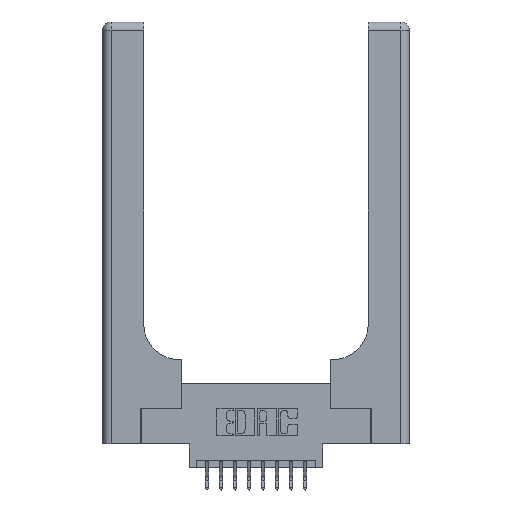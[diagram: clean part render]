
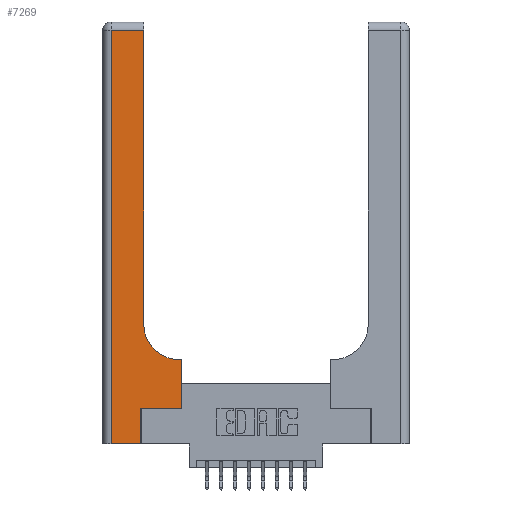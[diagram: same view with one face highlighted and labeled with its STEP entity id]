
A CAD part, top view. The second image highlights one B-rep face of the part: STEP entity #7269.
In plain terms, the highlighted planar face has unit normal (0, 0, 1).
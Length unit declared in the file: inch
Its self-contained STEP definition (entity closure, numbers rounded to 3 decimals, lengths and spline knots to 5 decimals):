
#210 = ORIENTED_EDGE ( 'NONE', *, *, #8994, .T. ) ;
#635 = CARTESIAN_POINT ( 'NONE',  ( 0.06, 0., 0.37 ) ) ;
#805 = EDGE_LOOP ( 'NONE', ( #210, #2820, #14824, #8057, #10947, #8593, #8192, #9050, #6819 ) ) ;
#823 = VERTEX_POINT ( 'NONE', #1749 ) ;
#869 = VERTEX_POINT ( 'NONE', #13013 ) ;
#1157 = CARTESIAN_POINT ( 'NONE',  ( 0.06, 3., 0.37 ) ) ;
#1540 = CARTESIAN_POINT ( 'NONE',  ( 0.269, 0.25, 0.37 ) ) ;
#1749 = CARTESIAN_POINT ( 'NONE',  ( 0.06, 2.94, 0.37 ) ) ;
#1825 = CARTESIAN_POINT ( 'NONE',  ( 0.269, 0.25, 0.37 ) ) ;
#2084 = CARTESIAN_POINT ( 'NONE',  ( 0.2915, 3., 0.37 ) ) ;
#2417 = DIRECTION ( 'NONE',  ( 1., 0., 0. ) ) ;
#2820 = ORIENTED_EDGE ( 'NONE', *, *, #3754, .T. ) ;
#2940 = VECTOR ( 'NONE', #7487, 39.37008 ) ;
#3478 = EDGE_CURVE ( 'NONE', #10670, #12525, #8065, .T. ) ;
#3628 = DIRECTION ( 'NONE',  ( -1., 0., 0. ) ) ;
#3647 = FACE_OUTER_BOUND ( 'NONE', #805, .T. ) ;
#3754 = EDGE_CURVE ( 'NONE', #12911, #823, #10224, .T. ) ;
#4066 = DIRECTION ( 'NONE',  ( -1., 0., 0. ) ) ;
#4224 = CARTESIAN_POINT ( 'NONE',  ( 0.269, 0., 0.37 ) ) ;
#4367 = VECTOR ( 'NONE', #3628, 39.37008 ) ;
#4794 = CARTESIAN_POINT ( 'NONE',  ( 0.2915, 0.6, 0.37 ) ) ;
#4896 = LINE ( 'NONE', #1157, #8446 ) ;
#5685 = VERTEX_POINT ( 'NONE', #9725 ) ;
#6125 = VECTOR ( 'NONE', #9954, 39.37008 ) ;
#6624 = DIRECTION ( 'NONE',  ( 0., 1., 0. ) ) ;
#6746 = CARTESIAN_POINT ( 'NONE',  ( 0., 2.94, 0.37 ) ) ;
#6755 = VECTOR ( 'NONE', #6624, 39.37008 ) ;
#6819 = ORIENTED_EDGE ( 'NONE', *, *, #9797, .T. ) ;
#7011 = DIRECTION ( 'NONE',  ( 0., 0., -1. ) ) ;
#7060 = CARTESIAN_POINT ( 'NONE',  ( 0.5585, 0.25, 0.37 ) ) ;
#7222 = DIRECTION ( 'NONE',  ( 0., 1., 0. ) ) ;
#7269 = ADVANCED_FACE ( 'NONE', ( #3647 ), #11799, .F. ) ;
#7487 = DIRECTION ( 'NONE',  ( 1., 0., 0. ) ) ;
#7496 = CIRCLE ( 'NONE', #7556, 0.25 ) ;
#7556 = AXIS2_PLACEMENT_3D ( 'NONE', #14958, #9977, #2417 ) ;
#8057 = ORIENTED_EDGE ( 'NONE', *, *, #15760, .T. ) ;
#8065 = LINE ( 'NONE', #1540, #2940 ) ;
#8192 = ORIENTED_EDGE ( 'NONE', *, *, #13709, .T. ) ;
#8216 = VERTEX_POINT ( 'NONE', #12868 ) ;
#8236 = EDGE_CURVE ( 'NONE', #869, #10670, #15256, .T. ) ;
#8339 = CARTESIAN_POINT ( 'NONE',  ( 0., 3., 0.37 ) ) ;
#8442 = DIRECTION ( 'NONE',  ( -1., 0., 0. ) ) ;
#8446 = VECTOR ( 'NONE', #8690, 39.37008 ) ;
#8593 = ORIENTED_EDGE ( 'NONE', *, *, #3478, .T. ) ;
#8606 = AXIS2_PLACEMENT_3D ( 'NONE', #8339, #7011, #8442 ) ;
#8690 = DIRECTION ( 'NONE',  ( 0., -1., 0. ) ) ;
#8994 = EDGE_CURVE ( 'NONE', #8216, #12911, #10885, .T. ) ;
#9050 = ORIENTED_EDGE ( 'NONE', *, *, #10193, .T. ) ;
#9725 = CARTESIAN_POINT ( 'NONE',  ( 0.5585, 0.6, 0.37 ) ) ;
#9797 = EDGE_CURVE ( 'NONE', #10331, #8216, #7496, .T. ) ;
#9954 = DIRECTION ( 'NONE',  ( 0., 1., 0. ) ) ;
#9977 = DIRECTION ( 'NONE',  ( 0., 0., -1. ) ) ;
#10193 = EDGE_CURVE ( 'NONE', #5685, #10331, #13441, .T. ) ;
#10224 = LINE ( 'NONE', #6746, #14786 ) ;
#10331 = VERTEX_POINT ( 'NONE', #13862 ) ;
#10670 = VERTEX_POINT ( 'NONE', #1825 ) ;
#10713 = LINE ( 'NONE', #12069, #15673 ) ;
#10872 = DIRECTION ( 'NONE',  ( 1., 0., 0. ) ) ;
#10885 = LINE ( 'NONE', #2084, #6125 ) ;
#10947 = ORIENTED_EDGE ( 'NONE', *, *, #8236, .T. ) ;
#11401 = VERTEX_POINT ( 'NONE', #635 ) ;
#11799 = PLANE ( 'NONE',  #8606 ) ;
#12069 = CARTESIAN_POINT ( 'NONE',  ( 0., 0., 0.37 ) ) ;
#12147 = LINE ( 'NONE', #7060, #15317 ) ;
#12211 = EDGE_CURVE ( 'NONE', #823, #11401, #4896, .T. ) ;
#12525 = VERTEX_POINT ( 'NONE', #13104 ) ;
#12868 = CARTESIAN_POINT ( 'NONE',  ( 0.2915, 0.85, 0.37 ) ) ;
#12911 = VERTEX_POINT ( 'NONE', #16203 ) ;
#13013 = CARTESIAN_POINT ( 'NONE',  ( 0.269, 0., 0.37 ) ) ;
#13104 = CARTESIAN_POINT ( 'NONE',  ( 0.5585, 0.25, 0.37 ) ) ;
#13441 = LINE ( 'NONE', #4794, #4367 ) ;
#13709 = EDGE_CURVE ( 'NONE', #12525, #5685, #12147, .T. ) ;
#13862 = CARTESIAN_POINT ( 'NONE',  ( 0.5415, 0.6, 0.37 ) ) ;
#14786 = VECTOR ( 'NONE', #4066, 39.37008 ) ;
#14824 = ORIENTED_EDGE ( 'NONE', *, *, #12211, .T. ) ;
#14958 = CARTESIAN_POINT ( 'NONE',  ( 0.5415, 0.85, 0.37 ) ) ;
#15256 = LINE ( 'NONE', #4224, #6755 ) ;
#15317 = VECTOR ( 'NONE', #7222, 39.37008 ) ;
#15673 = VECTOR ( 'NONE', #10872, 39.37008 ) ;
#15760 = EDGE_CURVE ( 'NONE', #11401, #869, #10713, .T. ) ;
#16203 = CARTESIAN_POINT ( 'NONE',  ( 0.2915, 2.94, 0.37 ) ) ;
